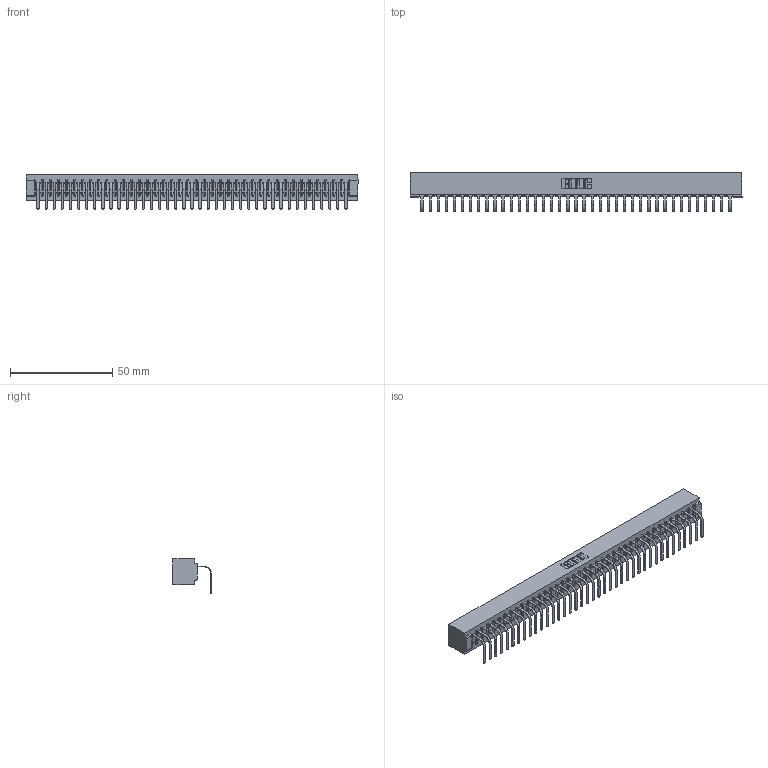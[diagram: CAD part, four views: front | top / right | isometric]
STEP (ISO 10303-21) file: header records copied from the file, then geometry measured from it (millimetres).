
FILE_DESCRIPTION (( 'STEP AP203' ), '1' );
FILE_NAME ('357-039-458-101.STEP', '2022-07-18T19:54:57', ( '' ), ( '' ), 'SwSTEP 2.0', 'SolidWorks 2020', '' );
FILE_SCHEMA (( 'CONFIG_CONTROL_DESIGN' ));
Length unit declared in the file: inch
Products named in the file (3): 357-039-458-101; 307 Part_No Mounting Lugs; 307-290-001_558 - 2 (Single)
Assembly tree (40 placements, depth 2):
  357-039-458-101
    307 Part_No Mounting Lugs
    307-290-001_558 - 2 (Single)  x39
Bounding box: 162.41 x 18.78 x 16.8 mm (x, y, z)
Volume: 17512.7 mm3; surface area: 19690.2 mm2
Topology: 40 solids, 40 shells, 2490 faces, 7085 edges, 4562 vertices
Faces by surface type: plane 1587, cylinder 823, sphere 80
Entity records: 33630 total; most frequent: CARTESIAN_POINT 5664, ORIENTED_EDGE 5650, DIRECTION 5509, EDGE_CURVE 2825, LINE 2167, VECTOR 2167, VERTEX_POINT 1826, AXIS2_PLACEMENT_3D 1671
